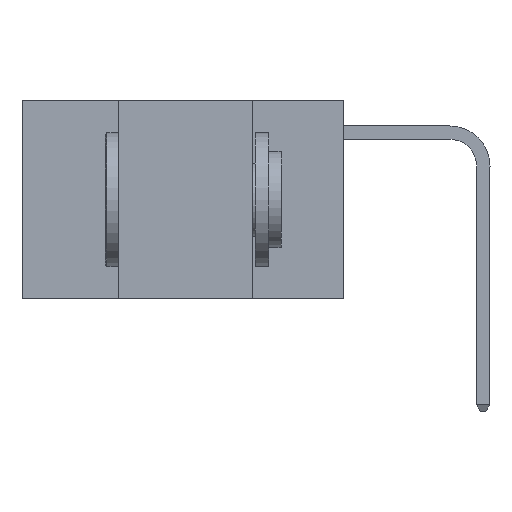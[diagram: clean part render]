
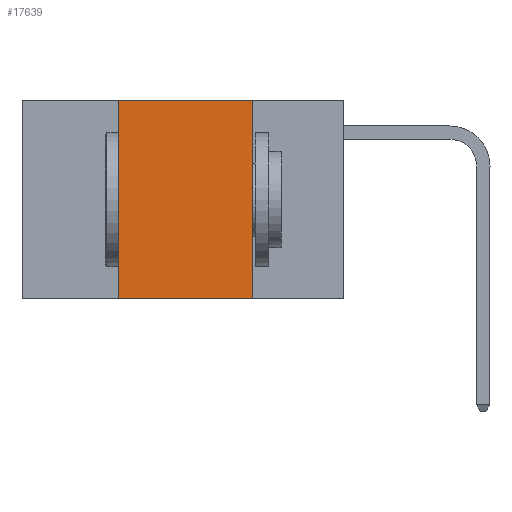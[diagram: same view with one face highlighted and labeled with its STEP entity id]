
A CAD part, left-side view. The second image highlights one B-rep face of the part: STEP entity #17639.
In plain terms, the highlighted planar face has unit normal (-1, 0, 0).
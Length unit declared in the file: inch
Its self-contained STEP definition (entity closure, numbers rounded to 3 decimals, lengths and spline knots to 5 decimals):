
#45 = VERTEX_POINT ( 'NONE', #14704 ) ;
#154 = DIRECTION ( 'NONE',  ( 1., 0., 0. ) ) ;
#221 = ORIENTED_EDGE ( 'NONE', *, *, #2796, .T. ) ;
#830 = DIRECTION ( 'NONE',  ( 0., 0., 1. ) ) ;
#1697 = CARTESIAN_POINT ( 'NONE',  ( 0., 0.42, 0. ) ) ;
#2796 = EDGE_CURVE ( 'NONE', #45, #19050, #15081, .T. ) ;
#3846 = CARTESIAN_POINT ( 'NONE',  ( 0., 0.6, 0. ) ) ;
#5169 = EDGE_CURVE ( 'NONE', #45, #15918, #21297, .T. ) ;
#6180 = EDGE_CURVE ( 'NONE', #16757, #19050, #23411, .T. ) ;
#8339 = ORIENTED_EDGE ( 'NONE', *, *, #5169, .F. ) ;
#8973 = CARTESIAN_POINT ( 'NONE',  ( 0., 0.17, 0. ) ) ;
#9484 = VECTOR ( 'NONE', #24625, 39.37008 ) ;
#10784 = PLANE ( 'NONE',  #18033 ) ;
#12415 = LINE ( 'NONE', #3846, #18017 ) ;
#13747 = CARTESIAN_POINT ( 'NONE',  ( 0., 0.17, -0.37 ) ) ;
#14704 = CARTESIAN_POINT ( 'NONE',  ( 0., 0.42, -0.37 ) ) ;
#15000 = DIRECTION ( 'NONE',  ( 0., 0., -1. ) ) ;
#15081 = LINE ( 'NONE', #22509, #9484 ) ;
#15918 = VERTEX_POINT ( 'NONE', #1697 ) ;
#16185 = EDGE_LOOP ( 'NONE', ( #18756, #25301, #8339, #221 ) ) ;
#16757 = VERTEX_POINT ( 'NONE', #17466 ) ;
#17126 = VECTOR ( 'NONE', #23745, 39.37008 ) ;
#17466 = CARTESIAN_POINT ( 'NONE',  ( 0., 0.17, 0. ) ) ;
#17639 = ADVANCED_FACE ( 'NONE', ( #18990 ), #10784, .F. ) ;
#17772 = CARTESIAN_POINT ( 'NONE',  ( 0., 0.42, 0. ) ) ;
#18017 = VECTOR ( 'NONE', #18612, 39.37008 ) ;
#18033 = AXIS2_PLACEMENT_3D ( 'NONE', #25548, #154, #15000 ) ;
#18612 = DIRECTION ( 'NONE',  ( 0., -1., 0. ) ) ;
#18756 = ORIENTED_EDGE ( 'NONE', *, *, #6180, .F. ) ;
#18990 = FACE_OUTER_BOUND ( 'NONE', #16185, .T. ) ;
#19050 = VERTEX_POINT ( 'NONE', #13747 ) ;
#21297 = LINE ( 'NONE', #17772, #26887 ) ;
#21379 = EDGE_CURVE ( 'NONE', #15918, #16757, #12415, .T. ) ;
#22509 = CARTESIAN_POINT ( 'NONE',  ( 0., 0.6, -0.37 ) ) ;
#23411 = LINE ( 'NONE', #8973, #17126 ) ;
#23745 = DIRECTION ( 'NONE',  ( 0., 0., -1. ) ) ;
#24625 = DIRECTION ( 'NONE',  ( 0., -1., 0. ) ) ;
#25301 = ORIENTED_EDGE ( 'NONE', *, *, #21379, .F. ) ;
#25548 = CARTESIAN_POINT ( 'NONE',  ( 0., 0.6, 0. ) ) ;
#26887 = VECTOR ( 'NONE', #830, 39.37008 ) ;
